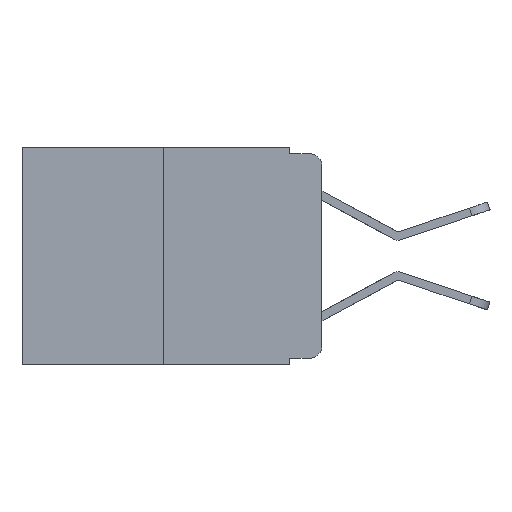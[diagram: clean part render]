
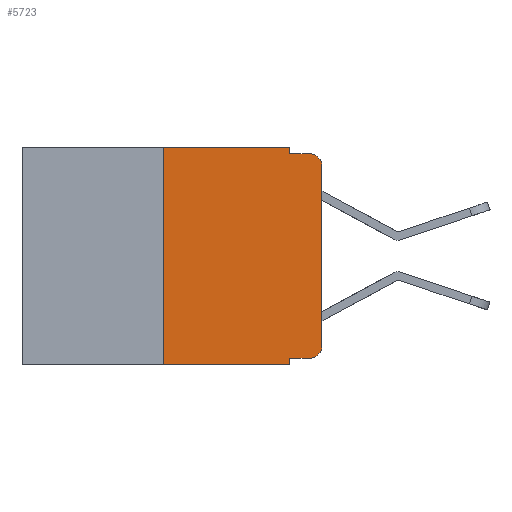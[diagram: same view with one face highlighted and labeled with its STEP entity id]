
A CAD part, left-side view. The second image highlights one B-rep face of the part: STEP entity #5723.
In plain terms, the highlighted planar face has unit normal (-1, 0, 0).
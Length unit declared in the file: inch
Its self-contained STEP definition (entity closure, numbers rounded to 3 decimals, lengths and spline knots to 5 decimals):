
#947 = VECTOR ( 'NONE', #4125, 39.37008 ) ;
#995 = VERTEX_POINT ( 'NONE', #6638 ) ;
#1258 = VECTOR ( 'NONE', #2786, 39.37008 ) ;
#1340 = VECTOR ( 'NONE', #3180, 39.37008 ) ;
#1392 = LINE ( 'NONE', #8136, #947 ) ;
#1656 = VERTEX_POINT ( 'NONE', #9412 ) ;
#1725 = EDGE_CURVE ( 'NONE', #995, #9548, #5525, .T. ) ;
#1778 = CARTESIAN_POINT ( 'NONE',  ( 0., 0.051, -0.343 ) ) ;
#1779 = DIRECTION ( 'NONE',  ( 0., 0., 1. ) ) ;
#1801 = CARTESIAN_POINT ( 'NONE',  ( 0., 0.02, -0.03 ) ) ;
#1887 = DIRECTION ( 'NONE',  ( 0., -1., 0. ) ) ;
#1904 = ORIENTED_EDGE ( 'NONE', *, *, #1725, .T. ) ;
#1964 = EDGE_CURVE ( 'NONE', #1656, #6391, #2553, .T. ) ;
#2144 = CARTESIAN_POINT ( 'NONE',  ( 0., 0.25, 0. ) ) ;
#2277 = DIRECTION ( 'NONE',  ( 0., 0., -1. ) ) ;
#2553 = LINE ( 'NONE', #16034, #15453 ) ;
#2708 = VECTOR ( 'NONE', #4060, 39.37008 ) ;
#2714 = VERTEX_POINT ( 'NONE', #3828 ) ;
#2786 = DIRECTION ( 'NONE',  ( 0., -1., 0. ) ) ;
#2816 = ORIENTED_EDGE ( 'NONE', *, *, #8662, .F. ) ;
#3180 = DIRECTION ( 'NONE',  ( 0., -1., 0. ) ) ;
#3184 = DIRECTION ( 'NONE',  ( 0., 0., -1. ) ) ;
#3828 = CARTESIAN_POINT ( 'NONE',  ( 0., 0., -0.03 ) ) ;
#4060 = DIRECTION ( 'NONE',  ( 0., 0., -1. ) ) ;
#4125 = DIRECTION ( 'NONE',  ( 0., 0., -1. ) ) ;
#4454 = LINE ( 'NONE', #11925, #1258 ) ;
#5100 = EDGE_CURVE ( 'NONE', #8358, #8478, #5460, .T. ) ;
#5460 = LINE ( 'NONE', #7831, #5890 ) ;
#5525 = CIRCLE ( 'NONE', #11436, 0.02 ) ;
#5723 = ADVANCED_FACE ( 'NONE', ( #12418 ), #15615, .F. ) ;
#5847 = CARTESIAN_POINT ( 'NONE',  ( 0., 0., 0. ) ) ;
#5890 = VECTOR ( 'NONE', #8422, 39.37008 ) ;
#5920 = CARTESIAN_POINT ( 'NONE',  ( 0., 0.473, -0.343 ) ) ;
#6305 = LINE ( 'NONE', #9797, #2708 ) ;
#6391 = VERTEX_POINT ( 'NONE', #8626 ) ;
#6405 = VECTOR ( 'NONE', #11612, 39.37008 ) ;
#6638 = CARTESIAN_POINT ( 'NONE',  ( 0., 0.02, -0.333 ) ) ;
#6943 = EDGE_LOOP ( 'NONE', ( #15911, #9378, #8909, #16292, #8802, #8787, #15631, #2816, #7674, #1904 ) ) ;
#7220 = EDGE_CURVE ( 'NONE', #8475, #995, #4454, .T. ) ;
#7540 = AXIS2_PLACEMENT_3D ( 'NONE', #8363, #16366, #2277 ) ;
#7674 = ORIENTED_EDGE ( 'NONE', *, *, #7220, .T. ) ;
#7831 = CARTESIAN_POINT ( 'NONE',  ( 0., 0.473, 0. ) ) ;
#8136 = CARTESIAN_POINT ( 'NONE',  ( 0., 0.051, 0. ) ) ;
#8358 = VERTEX_POINT ( 'NONE', #2144 ) ;
#8363 = CARTESIAN_POINT ( 'NONE',  ( 0., 0.473, 0. ) ) ;
#8422 = DIRECTION ( 'NONE',  ( 0., -1., 0. ) ) ;
#8475 = VERTEX_POINT ( 'NONE', #12093 ) ;
#8478 = VERTEX_POINT ( 'NONE', #11858 ) ;
#8558 = LINE ( 'NONE', #5920, #1340 ) ;
#8626 = CARTESIAN_POINT ( 'NONE',  ( 0., 0.02, -0.01 ) ) ;
#8662 = EDGE_CURVE ( 'NONE', #8475, #12321, #6305, .T. ) ;
#8753 = CARTESIAN_POINT ( 'NONE',  ( 0., 0., -0.313 ) ) ;
#8787 = ORIENTED_EDGE ( 'NONE', *, *, #11167, .F. ) ;
#8802 = ORIENTED_EDGE ( 'NONE', *, *, #5100, .F. ) ;
#8909 = ORIENTED_EDGE ( 'NONE', *, *, #1964, .F. ) ;
#9111 = CARTESIAN_POINT ( 'NONE',  ( 0., 0.25, 0. ) ) ;
#9117 = VECTOR ( 'NONE', #1779, 39.37008 ) ;
#9378 = ORIENTED_EDGE ( 'NONE', *, *, #11676, .T. ) ;
#9412 = CARTESIAN_POINT ( 'NONE',  ( 0., 0.051, -0.01 ) ) ;
#9548 = VERTEX_POINT ( 'NONE', #8753 ) ;
#9797 = CARTESIAN_POINT ( 'NONE',  ( 0., 0.051, 0. ) ) ;
#9970 = EDGE_CURVE ( 'NONE', #15423, #12321, #8558, .T. ) ;
#10300 = LINE ( 'NONE', #9111, #6405 ) ;
#10654 = CARTESIAN_POINT ( 'NONE',  ( 0., 0.02, -0.313 ) ) ;
#11076 = DIRECTION ( 'NONE',  ( -1., 0., 0. ) ) ;
#11167 = EDGE_CURVE ( 'NONE', #15423, #8358, #10300, .T. ) ;
#11390 = DIRECTION ( 'NONE',  ( -1., 0., 0. ) ) ;
#11436 = AXIS2_PLACEMENT_3D ( 'NONE', #10654, #11390, #11944 ) ;
#11612 = DIRECTION ( 'NONE',  ( 0., 0., 1. ) ) ;
#11676 = EDGE_CURVE ( 'NONE', #2714, #6391, #12104, .T. ) ;
#11858 = CARTESIAN_POINT ( 'NONE',  ( 0., 0.051, 0. ) ) ;
#11925 = CARTESIAN_POINT ( 'NONE',  ( 0., 0.051, -0.333 ) ) ;
#11944 = DIRECTION ( 'NONE',  ( 0., 0., -1. ) ) ;
#12093 = CARTESIAN_POINT ( 'NONE',  ( 0., 0.051, -0.333 ) ) ;
#12104 = CIRCLE ( 'NONE', #14569, 0.02 ) ;
#12281 = CARTESIAN_POINT ( 'NONE',  ( 0., 0.25, -0.343 ) ) ;
#12321 = VERTEX_POINT ( 'NONE', #1778 ) ;
#12362 = LINE ( 'NONE', #5847, #9117 ) ;
#12418 = FACE_OUTER_BOUND ( 'NONE', #6943, .T. ) ;
#12744 = EDGE_CURVE ( 'NONE', #8478, #1656, #1392, .T. ) ;
#14569 = AXIS2_PLACEMENT_3D ( 'NONE', #1801, #11076, #3184 ) ;
#14673 = EDGE_CURVE ( 'NONE', #9548, #2714, #12362, .T. ) ;
#15423 = VERTEX_POINT ( 'NONE', #12281 ) ;
#15453 = VECTOR ( 'NONE', #1887, 39.37008 ) ;
#15615 = PLANE ( 'NONE',  #7540 ) ;
#15631 = ORIENTED_EDGE ( 'NONE', *, *, #9970, .T. ) ;
#15911 = ORIENTED_EDGE ( 'NONE', *, *, #14673, .T. ) ;
#16034 = CARTESIAN_POINT ( 'NONE',  ( 0., 0.051, -0.01 ) ) ;
#16292 = ORIENTED_EDGE ( 'NONE', *, *, #12744, .F. ) ;
#16366 = DIRECTION ( 'NONE',  ( 1., 0., 0. ) ) ;
